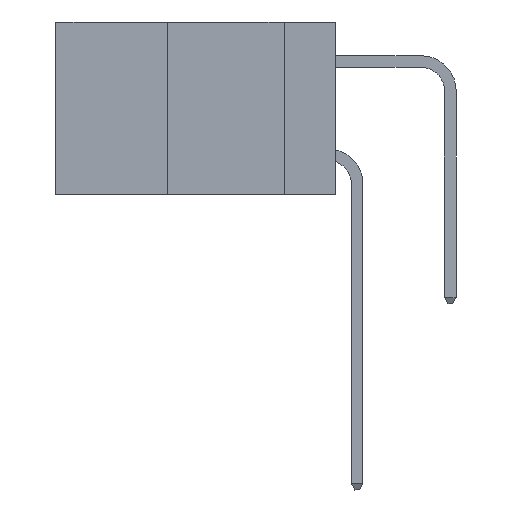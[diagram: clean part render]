
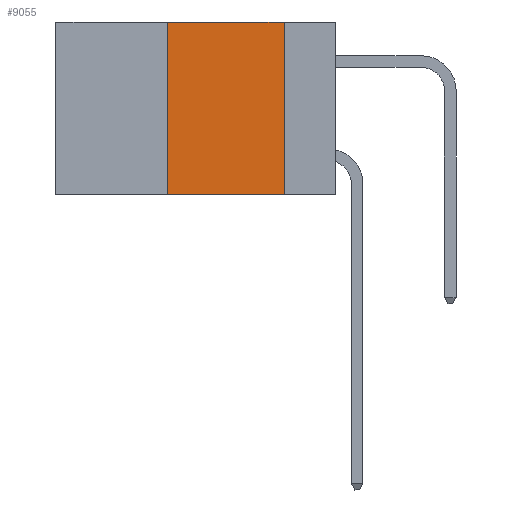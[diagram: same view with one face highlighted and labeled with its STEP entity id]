
A CAD part, left-side view. The second image highlights one B-rep face of the part: STEP entity #9055.
In plain terms, the highlighted planar face has unit normal (-1, 0, 0).
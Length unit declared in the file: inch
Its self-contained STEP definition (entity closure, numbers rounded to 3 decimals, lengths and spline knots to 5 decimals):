
#675 = VERTEX_POINT ( 'NONE', #18990 ) ;
#1642 = EDGE_LOOP ( 'NONE', ( #3919, #5088, #14057, #6075 ) ) ;
#1696 = EDGE_CURVE ( 'NONE', #5745, #14635, #13625, .T. ) ;
#2126 = EDGE_CURVE ( 'NONE', #14635, #9485, #14443, .T. ) ;
#2537 = LINE ( 'NONE', #3418, #14552 ) ;
#2559 = CARTESIAN_POINT ( 'NONE',  ( 0., 0.36, -0.37 ) ) ;
#3418 = CARTESIAN_POINT ( 'NONE',  ( 0., 0.6, -0.37 ) ) ;
#3600 = CARTESIAN_POINT ( 'NONE',  ( 0., 0.6, 0. ) ) ;
#3919 = ORIENTED_EDGE ( 'NONE', *, *, #4130, .F. ) ;
#4102 = CARTESIAN_POINT ( 'NONE',  ( 0., 0.11, 0. ) ) ;
#4123 = CARTESIAN_POINT ( 'NONE',  ( 0., 0.11, 0. ) ) ;
#4130 = EDGE_CURVE ( 'NONE', #9485, #675, #10212, .T. ) ;
#4572 = PLANE ( 'NONE',  #6141 ) ;
#5020 = DIRECTION ( 'NONE',  ( 0., -1., 0. ) ) ;
#5088 = ORIENTED_EDGE ( 'NONE', *, *, #2126, .F. ) ;
#5745 = VERTEX_POINT ( 'NONE', #2559 ) ;
#6075 = ORIENTED_EDGE ( 'NONE', *, *, #6131, .T. ) ;
#6131 = EDGE_CURVE ( 'NONE', #5745, #675, #2537, .T. ) ;
#6136 = DIRECTION ( 'NONE',  ( 0., 0., -1. ) ) ;
#6141 = AXIS2_PLACEMENT_3D ( 'NONE', #20155, #15508, #6136 ) ;
#9055 = ADVANCED_FACE ( 'NONE', ( #18624 ), #4572, .F. ) ;
#9425 = VECTOR ( 'NONE', #15035, 39.37008 ) ;
#9485 = VERTEX_POINT ( 'NONE', #4123 ) ;
#10145 = DIRECTION ( 'NONE',  ( 0., -1., 0. ) ) ;
#10158 = CARTESIAN_POINT ( 'NONE',  ( 0., 0.36, 0. ) ) ;
#10212 = LINE ( 'NONE', #4102, #18078 ) ;
#11900 = CARTESIAN_POINT ( 'NONE',  ( 0., 0.36, 0. ) ) ;
#13516 = DIRECTION ( 'NONE',  ( 0., 0., -1. ) ) ;
#13625 = LINE ( 'NONE', #11900, #9425 ) ;
#14057 = ORIENTED_EDGE ( 'NONE', *, *, #1696, .F. ) ;
#14443 = LINE ( 'NONE', #3600, #18134 ) ;
#14552 = VECTOR ( 'NONE', #5020, 39.37008 ) ;
#14635 = VERTEX_POINT ( 'NONE', #10158 ) ;
#15035 = DIRECTION ( 'NONE',  ( 0., 0., 1. ) ) ;
#15508 = DIRECTION ( 'NONE',  ( 1., 0., 0. ) ) ;
#18078 = VECTOR ( 'NONE', #13516, 39.37008 ) ;
#18134 = VECTOR ( 'NONE', #10145, 39.37008 ) ;
#18624 = FACE_OUTER_BOUND ( 'NONE', #1642, .T. ) ;
#18990 = CARTESIAN_POINT ( 'NONE',  ( 0., 0.11, -0.37 ) ) ;
#20155 = CARTESIAN_POINT ( 'NONE',  ( 0., 0.6, 0. ) ) ;
